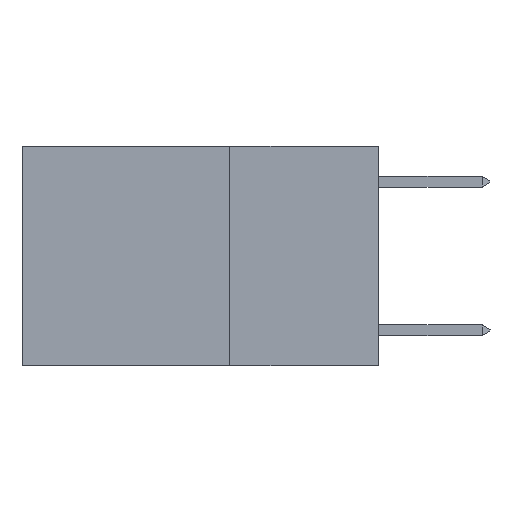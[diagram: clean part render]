
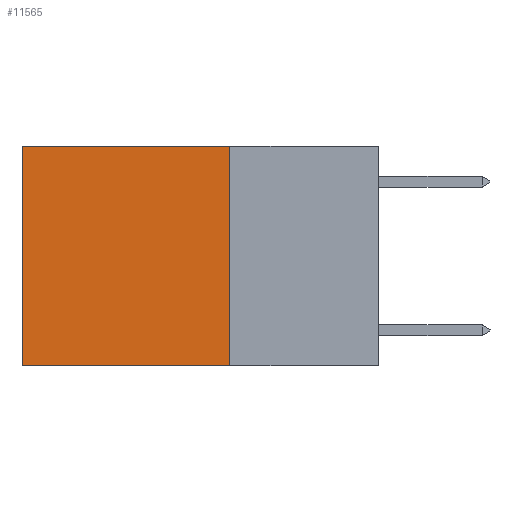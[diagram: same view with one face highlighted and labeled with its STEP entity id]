
A CAD part, left-side view. The second image highlights one B-rep face of the part: STEP entity #11565.
In plain terms, the highlighted planar face has unit normal (-1, 0, 0).
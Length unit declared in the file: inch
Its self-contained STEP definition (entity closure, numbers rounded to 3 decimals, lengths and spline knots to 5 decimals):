
#551 = DIRECTION ( 'NONE',  ( 1., 0., 0. ) ) ;
#596 = VERTEX_POINT ( 'NONE', #8652 ) ;
#691 = DIRECTION ( 'NONE',  ( 0., 1., 0. ) ) ;
#1226 = VECTOR ( 'NONE', #16148, 39.37008 ) ;
#1740 = EDGE_CURVE ( 'NONE', #7818, #9564, #5060, .T. ) ;
#2416 = ORIENTED_EDGE ( 'NONE', *, *, #3410, .F. ) ;
#3335 = VECTOR ( 'NONE', #691, 39.37008 ) ;
#3410 = EDGE_CURVE ( 'NONE', #9564, #12225, #6400, .T. ) ;
#3967 = VECTOR ( 'NONE', #11362, 39.37008 ) ;
#4658 = EDGE_LOOP ( 'NONE', ( #15879, #2416, #14095, #12368 ) ) ;
#5060 = LINE ( 'NONE', #13590, #1226 ) ;
#5645 = FACE_OUTER_BOUND ( 'NONE', #4658, .T. ) ;
#6400 = LINE ( 'NONE', #15551, #9330 ) ;
#6961 = CARTESIAN_POINT ( 'NONE',  ( 0.2625, 0.25, -0.37 ) ) ;
#6995 = AXIS2_PLACEMENT_3D ( 'NONE', #9368, #551, #9422 ) ;
#7818 = VERTEX_POINT ( 'NONE', #14818 ) ;
#8181 = PLANE ( 'NONE',  #6995 ) ;
#8322 = CARTESIAN_POINT ( 'NONE',  ( 0.2625, 0.25, 0. ) ) ;
#8652 = CARTESIAN_POINT ( 'NONE',  ( 0.2625, 0.6, 0. ) ) ;
#8887 = CARTESIAN_POINT ( 'NONE',  ( 0.2625, 0.6, 0. ) ) ;
#9330 = VECTOR ( 'NONE', #10542, 39.37008 ) ;
#9368 = CARTESIAN_POINT ( 'NONE',  ( 0.2625, 0.25, 0. ) ) ;
#9422 = DIRECTION ( 'NONE',  ( 0., 0., -1. ) ) ;
#9564 = VERTEX_POINT ( 'NONE', #6961 ) ;
#9623 = EDGE_CURVE ( 'NONE', #7818, #596, #10021, .T. ) ;
#10021 = LINE ( 'NONE', #8322, #3335 ) ;
#10542 = DIRECTION ( 'NONE',  ( 0., 1., 0. ) ) ;
#11362 = DIRECTION ( 'NONE',  ( 0., 0., -1. ) ) ;
#11565 = ADVANCED_FACE ( 'NONE', ( #5645 ), #8181, .F. ) ;
#12225 = VERTEX_POINT ( 'NONE', #13093 ) ;
#12368 = ORIENTED_EDGE ( 'NONE', *, *, #9623, .T. ) ;
#13093 = CARTESIAN_POINT ( 'NONE',  ( 0.2625, 0.6, -0.37 ) ) ;
#13590 = CARTESIAN_POINT ( 'NONE',  ( 0.2625, 0.25, 0. ) ) ;
#13927 = EDGE_CURVE ( 'NONE', #596, #12225, #13947, .T. ) ;
#13947 = LINE ( 'NONE', #8887, #3967 ) ;
#14095 = ORIENTED_EDGE ( 'NONE', *, *, #1740, .F. ) ;
#14818 = CARTESIAN_POINT ( 'NONE',  ( 0.2625, 0.25, 0. ) ) ;
#15551 = CARTESIAN_POINT ( 'NONE',  ( 0.2625, 0.25, -0.37 ) ) ;
#15879 = ORIENTED_EDGE ( 'NONE', *, *, #13927, .T. ) ;
#16148 = DIRECTION ( 'NONE',  ( 0., 0., -1. ) ) ;
